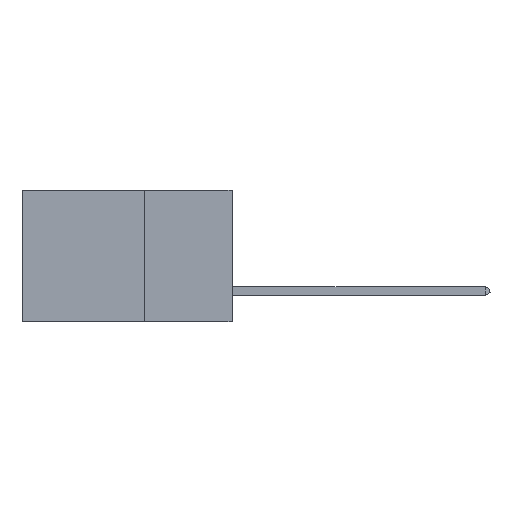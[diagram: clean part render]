
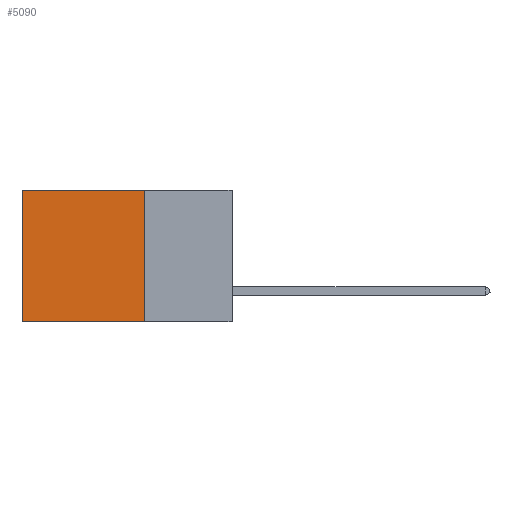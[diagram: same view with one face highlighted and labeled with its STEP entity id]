
A CAD part, left-side view. The second image highlights one B-rep face of the part: STEP entity #5090.
In plain terms, the highlighted planar face has unit normal (-1, 0, 0).
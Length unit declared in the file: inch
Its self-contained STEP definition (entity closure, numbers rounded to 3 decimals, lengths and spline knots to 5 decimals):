
#678 = DIRECTION ( 'NONE',  ( 0., 0., -1. ) ) ;
#978 = LINE ( 'NONE', #16136, #7695 ) ;
#1967 = CARTESIAN_POINT ( 'NONE',  ( 0.2875, 0.25, -0.375 ) ) ;
#2340 = EDGE_CURVE ( 'NONE', #11478, #16568, #18298, .T. ) ;
#2473 = ORIENTED_EDGE ( 'NONE', *, *, #10323, .T. ) ;
#2502 = ORIENTED_EDGE ( 'NONE', *, *, #19348, .T. ) ;
#3278 = DIRECTION ( 'NONE',  ( 0., 0., -1. ) ) ;
#4055 = LINE ( 'NONE', #5037, #12083 ) ;
#4356 = VECTOR ( 'NONE', #678, 39.37008 ) ;
#4687 = DIRECTION ( 'NONE',  ( 1., 0., 0. ) ) ;
#5037 = CARTESIAN_POINT ( 'NONE',  ( 0.2875, 0.25, -0.375 ) ) ;
#5090 = ADVANCED_FACE ( 'NONE', ( #12135 ), #8198, .F. ) ;
#5506 = VERTEX_POINT ( 'NONE', #8948 ) ;
#5573 = VECTOR ( 'NONE', #13145, 39.37008 ) ;
#6507 = VERTEX_POINT ( 'NONE', #17050 ) ;
#7402 = AXIS2_PLACEMENT_3D ( 'NONE', #14560, #4687, #15881 ) ;
#7695 = VECTOR ( 'NONE', #20656, 39.37008 ) ;
#7801 = CARTESIAN_POINT ( 'NONE',  ( 0.2875, 0.25, -0.375 ) ) ;
#8198 = PLANE ( 'NONE',  #7402 ) ;
#8948 = CARTESIAN_POINT ( 'NONE',  ( 0.2875, 0.25, 0. ) ) ;
#10323 = EDGE_CURVE ( 'NONE', #6507, #16568, #12880, .T. ) ;
#10814 = CARTESIAN_POINT ( 'NONE',  ( 0.2875, 0.6, -0.375 ) ) ;
#11478 = VERTEX_POINT ( 'NONE', #7801 ) ;
#12083 = VECTOR ( 'NONE', #3278, 39.37008 ) ;
#12135 = FACE_OUTER_BOUND ( 'NONE', #20163, .T. ) ;
#12880 = LINE ( 'NONE', #16652, #4356 ) ;
#13145 = DIRECTION ( 'NONE',  ( 0., 1., 0. ) ) ;
#14560 = CARTESIAN_POINT ( 'NONE',  ( 0.2875, 0.25, -0.375 ) ) ;
#15528 = ORIENTED_EDGE ( 'NONE', *, *, #2340, .F. ) ;
#15881 = DIRECTION ( 'NONE',  ( 0., 0., -1. ) ) ;
#16136 = CARTESIAN_POINT ( 'NONE',  ( 0.2875, 0.25, 0. ) ) ;
#16568 = VERTEX_POINT ( 'NONE', #10814 ) ;
#16652 = CARTESIAN_POINT ( 'NONE',  ( 0.2875, 0.6, -0.375 ) ) ;
#16788 = EDGE_CURVE ( 'NONE', #5506, #11478, #4055, .T. ) ;
#17050 = CARTESIAN_POINT ( 'NONE',  ( 0.2875, 0.6, 0. ) ) ;
#18298 = LINE ( 'NONE', #1967, #5573 ) ;
#19348 = EDGE_CURVE ( 'NONE', #5506, #6507, #978, .T. ) ;
#19518 = ORIENTED_EDGE ( 'NONE', *, *, #16788, .F. ) ;
#20163 = EDGE_LOOP ( 'NONE', ( #2473, #15528, #19518, #2502 ) ) ;
#20656 = DIRECTION ( 'NONE',  ( 0., 1., 0. ) ) ;
